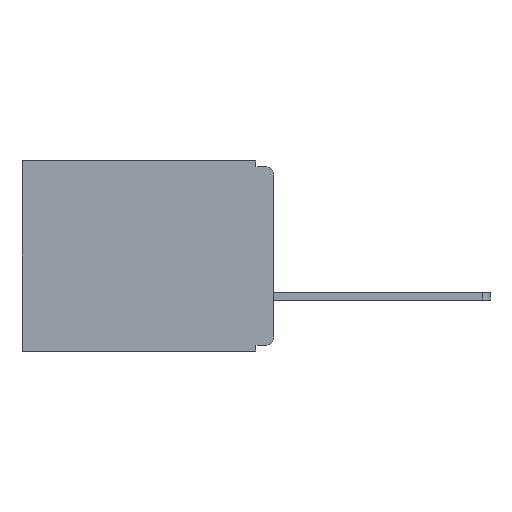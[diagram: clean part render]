
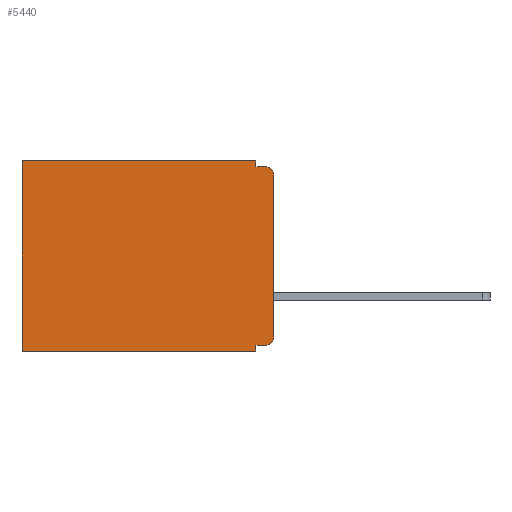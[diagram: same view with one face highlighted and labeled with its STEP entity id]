
A CAD part, left-side view. The second image highlights one B-rep face of the part: STEP entity #5440.
In plain terms, the highlighted planar face has unit normal (-1, 0, 0).
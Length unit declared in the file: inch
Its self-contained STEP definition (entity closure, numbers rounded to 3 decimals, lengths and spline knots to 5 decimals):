
#12 = ORIENTED_EDGE ( 'NONE', *, *, #11402, .F. ) ;
#53 = CARTESIAN_POINT ( 'NONE',  ( 0.3, 0., -0.01 ) ) ;
#100 = ORIENTED_EDGE ( 'NONE', *, *, #6324, .T. ) ;
#214 = DIRECTION ( 'NONE',  ( 0., -1., 0. ) ) ;
#309 = DIRECTION ( 'NONE',  ( 0., 1., 0. ) ) ;
#483 = ORIENTED_EDGE ( 'NONE', *, *, #7117, .T. ) ;
#605 = DIRECTION ( 'NONE',  ( 0., 0., -1. ) ) ;
#629 = ORIENTED_EDGE ( 'NONE', *, *, #2478, .F. ) ;
#741 = ORIENTED_EDGE ( 'NONE', *, *, #17628, .F. ) ;
#816 = ORIENTED_EDGE ( 'NONE', *, *, #13362, .F. ) ;
#896 = VERTEX_POINT ( 'NONE', #9611 ) ;
#1014 = DIRECTION ( 'NONE',  ( 0., 1., 0. ) ) ;
#1048 = ORIENTED_EDGE ( 'NONE', *, *, #9604, .T. ) ;
#1158 = CARTESIAN_POINT ( 'NONE',  ( 0.3, 0., -0.32 ) ) ;
#1569 = VERTEX_POINT ( 'NONE', #10428 ) ;
#1736 = CARTESIAN_POINT ( 'NONE',  ( 0.3, 0.031, 0. ) ) ;
#1864 = CARTESIAN_POINT ( 'NONE',  ( 0.3, 0., -0.33 ) ) ;
#2478 = EDGE_CURVE ( 'NONE', #1569, #896, #4649, .T. ) ;
#2826 = VERTEX_POINT ( 'NONE', #7883 ) ;
#3105 = VECTOR ( 'NONE', #309, 39.37008 ) ;
#3126 = VERTEX_POINT ( 'NONE', #6951 ) ;
#3222 = CARTESIAN_POINT ( 'NONE',  ( 0.3, 0.031, -0.32 ) ) ;
#3465 = EDGE_CURVE ( 'NONE', #13803, #10467, #10826, .T. ) ;
#3608 = CARTESIAN_POINT ( 'NONE',  ( 0.3, 0., -0.33 ) ) ;
#3856 = VERTEX_POINT ( 'NONE', #7850 ) ;
#3955 = ORIENTED_EDGE ( 'NONE', *, *, #11528, .F. ) ;
#4463 = DIRECTION ( 'NONE',  ( 0., 0., -1. ) ) ;
#4579 = CARTESIAN_POINT ( 'NONE',  ( 0.3, 0.015, -0.025 ) ) ;
#4649 = LINE ( 'NONE', #3608, #3105 ) ;
#4728 = CARTESIAN_POINT ( 'NONE',  ( 0.3, 0., -0.33 ) ) ;
#4839 = VERTEX_POINT ( 'NONE', #11531 ) ;
#5056 = DIRECTION ( 'NONE',  ( -1., 0., 0. ) ) ;
#5440 = ADVANCED_FACE ( 'NONE', ( #16180 ), #14787, .F. ) ;
#5676 = LINE ( 'NONE', #53, #5878 ) ;
#5878 = VECTOR ( 'NONE', #214, 39.37008 ) ;
#6324 = EDGE_CURVE ( 'NONE', #3126, #896, #11434, .T. ) ;
#6951 = CARTESIAN_POINT ( 'NONE',  ( 0.3, 0.437, 0. ) ) ;
#7009 = CIRCLE ( 'NONE', #16330, 0.015 ) ;
#7029 = DIRECTION ( 'NONE',  ( 0., 0., -1. ) ) ;
#7050 = DIRECTION ( 'NONE',  ( -1., 0., 0. ) ) ;
#7078 = CARTESIAN_POINT ( 'NONE',  ( 0.3, 0.015, -0.305 ) ) ;
#7117 = EDGE_CURVE ( 'NONE', #8601, #3126, #8365, .T. ) ;
#7350 = ORIENTED_EDGE ( 'NONE', *, *, #11690, .F. ) ;
#7639 = VERTEX_POINT ( 'NONE', #3222 ) ;
#7818 = CARTESIAN_POINT ( 'NONE',  ( 0.3, 0.015, -0.01 ) ) ;
#7850 = CARTESIAN_POINT ( 'NONE',  ( 0.3, 0.031, -0.01 ) ) ;
#7883 = CARTESIAN_POINT ( 'NONE',  ( 0.3, 0., -0.305 ) ) ;
#8302 = VECTOR ( 'NONE', #1014, 39.37008 ) ;
#8307 = LINE ( 'NONE', #1158, #8302 ) ;
#8350 = VECTOR ( 'NONE', #12249, 39.37008 ) ;
#8365 = LINE ( 'NONE', #12674, #8350 ) ;
#8601 = VERTEX_POINT ( 'NONE', #1736 ) ;
#9198 = CARTESIAN_POINT ( 'NONE',  ( 0.3, 0.031, 0. ) ) ;
#9349 = DIRECTION ( 'NONE',  ( 0., 0., -1. ) ) ;
#9604 = EDGE_CURVE ( 'NONE', #4839, #2826, #7009, .T. ) ;
#9611 = CARTESIAN_POINT ( 'NONE',  ( 0.3, 0.437, -0.33 ) ) ;
#10008 = CARTESIAN_POINT ( 'NONE',  ( 0.3, 0.437, -0.33 ) ) ;
#10428 = CARTESIAN_POINT ( 'NONE',  ( 0.3, 0.031, -0.33 ) ) ;
#10467 = VERTEX_POINT ( 'NONE', #7818 ) ;
#10826 = CIRCLE ( 'NONE', #14031, 0.015 ) ;
#11310 = VECTOR ( 'NONE', #13846, 39.37008 ) ;
#11402 = EDGE_CURVE ( 'NONE', #8601, #3856, #14402, .T. ) ;
#11434 = LINE ( 'NONE', #10008, #11310 ) ;
#11528 = EDGE_CURVE ( 'NONE', #13803, #2826, #13790, .T. ) ;
#11531 = CARTESIAN_POINT ( 'NONE',  ( 0.3, 0.015, -0.32 ) ) ;
#11690 = EDGE_CURVE ( 'NONE', #3856, #10467, #5676, .T. ) ;
#12249 = DIRECTION ( 'NONE',  ( 0., 1., 0. ) ) ;
#12674 = CARTESIAN_POINT ( 'NONE',  ( 0.3, 0., 0. ) ) ;
#13362 = EDGE_CURVE ( 'NONE', #4839, #7639, #8307, .T. ) ;
#13551 = DIRECTION ( 'NONE',  ( 0., 0., -1. ) ) ;
#13790 = LINE ( 'NONE', #4728, #13825 ) ;
#13803 = VERTEX_POINT ( 'NONE', #16596 ) ;
#13825 = VECTOR ( 'NONE', #4463, 39.37008 ) ;
#13846 = DIRECTION ( 'NONE',  ( 0., 0., -1. ) ) ;
#14013 = CARTESIAN_POINT ( 'NONE',  ( 0.3, 0.031, -0.33 ) ) ;
#14031 = AXIS2_PLACEMENT_3D ( 'NONE', #4579, #5056, #605 ) ;
#14254 = VECTOR ( 'NONE', #9349, 39.37008 ) ;
#14343 = VECTOR ( 'NONE', #13551, 39.37008 ) ;
#14402 = LINE ( 'NONE', #9198, #14254 ) ;
#14655 = LINE ( 'NONE', #14013, #14343 ) ;
#14787 = PLANE ( 'NONE',  #17184 ) ;
#15487 = DIRECTION ( 'NONE',  ( 1., 0., 0. ) ) ;
#15762 = DIRECTION ( 'NONE',  ( 0., 0., -1. ) ) ;
#16180 = FACE_OUTER_BOUND ( 'NONE', #17460, .T. ) ;
#16330 = AXIS2_PLACEMENT_3D ( 'NONE', #7078, #7050, #7029 ) ;
#16596 = CARTESIAN_POINT ( 'NONE',  ( 0.3, 0., -0.025 ) ) ;
#16739 = ORIENTED_EDGE ( 'NONE', *, *, #3465, .T. ) ;
#17184 = AXIS2_PLACEMENT_3D ( 'NONE', #1864, #15487, #15762 ) ;
#17460 = EDGE_LOOP ( 'NONE', ( #3955, #16739, #7350, #12, #483, #100, #629, #741, #816, #1048 ) ) ;
#17628 = EDGE_CURVE ( 'NONE', #7639, #1569, #14655, .T. ) ;
